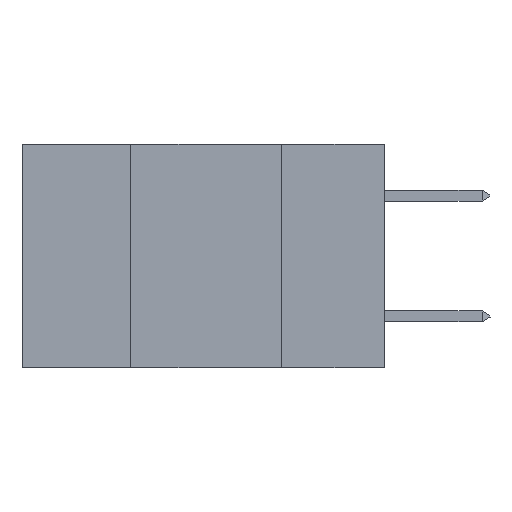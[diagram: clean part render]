
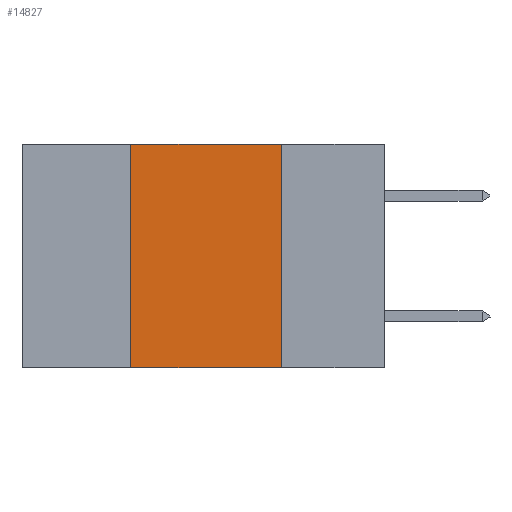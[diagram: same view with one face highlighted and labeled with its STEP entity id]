
A CAD part, left-side view. The second image highlights one B-rep face of the part: STEP entity #14827.
In plain terms, the highlighted planar face has unit normal (-1, 0, 0).
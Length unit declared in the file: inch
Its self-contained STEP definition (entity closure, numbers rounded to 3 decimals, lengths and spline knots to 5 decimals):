
#586 = ORIENTED_EDGE ( 'NONE', *, *, #3465, .F. ) ;
#590 = VERTEX_POINT ( 'NONE', #19543 ) ;
#3465 = EDGE_CURVE ( 'NONE', #14657, #19105, #22983, .T. ) ;
#3655 = VECTOR ( 'NONE', #4367, 39.37008 ) ;
#4367 = DIRECTION ( 'NONE',  ( 0., 0., 1. ) ) ;
#5887 = ORIENTED_EDGE ( 'NONE', *, *, #21849, .F. ) ;
#5935 = EDGE_CURVE ( 'NONE', #590, #14657, #8927, .T. ) ;
#6019 = AXIS2_PLACEMENT_3D ( 'NONE', #14275, #8492, #20450 ) ;
#7106 = LINE ( 'NONE', #9485, #13103 ) ;
#7917 = CARTESIAN_POINT ( 'NONE',  ( 0., 0.42, 0. ) ) ;
#8049 = CARTESIAN_POINT ( 'NONE',  ( 0., 0.42, 0. ) ) ;
#8144 = CARTESIAN_POINT ( 'NONE',  ( 0., 0.17, 0. ) ) ;
#8492 = DIRECTION ( 'NONE',  ( 1., 0., 0. ) ) ;
#8927 = LINE ( 'NONE', #7917, #3655 ) ;
#9079 = CARTESIAN_POINT ( 'NONE',  ( 0., 0.17, 0. ) ) ;
#9485 = CARTESIAN_POINT ( 'NONE',  ( 0., 0.6, -0.37 ) ) ;
#10886 = EDGE_LOOP ( 'NONE', ( #5887, #586, #18113, #23321 ) ) ;
#13103 = VECTOR ( 'NONE', #16216, 39.37008 ) ;
#14131 = FACE_OUTER_BOUND ( 'NONE', #10886, .T. ) ;
#14275 = CARTESIAN_POINT ( 'NONE',  ( 0., 0.6, 0. ) ) ;
#14657 = VERTEX_POINT ( 'NONE', #8049 ) ;
#14827 = ADVANCED_FACE ( 'NONE', ( #14131 ), #24485, .F. ) ;
#15045 = VERTEX_POINT ( 'NONE', #16403 ) ;
#15372 = DIRECTION ( 'NONE',  ( 0., 0., -1. ) ) ;
#16216 = DIRECTION ( 'NONE',  ( 0., -1., 0. ) ) ;
#16232 = DIRECTION ( 'NONE',  ( 0., -1., 0. ) ) ;
#16399 = VECTOR ( 'NONE', #15372, 39.37008 ) ;
#16403 = CARTESIAN_POINT ( 'NONE',  ( 0., 0.17, -0.37 ) ) ;
#17612 = VECTOR ( 'NONE', #16232, 39.37008 ) ;
#18113 = ORIENTED_EDGE ( 'NONE', *, *, #5935, .F. ) ;
#19105 = VERTEX_POINT ( 'NONE', #8144 ) ;
#19543 = CARTESIAN_POINT ( 'NONE',  ( 0., 0.42, -0.37 ) ) ;
#19889 = LINE ( 'NONE', #9079, #16399 ) ;
#20450 = DIRECTION ( 'NONE',  ( 0., 0., -1. ) ) ;
#21849 = EDGE_CURVE ( 'NONE', #19105, #15045, #19889, .T. ) ;
#22983 = LINE ( 'NONE', #24237, #17612 ) ;
#23321 = ORIENTED_EDGE ( 'NONE', *, *, #25782, .T. ) ;
#24237 = CARTESIAN_POINT ( 'NONE',  ( 0., 0.6, 0. ) ) ;
#24485 = PLANE ( 'NONE',  #6019 ) ;
#25782 = EDGE_CURVE ( 'NONE', #590, #15045, #7106, .T. ) ;
